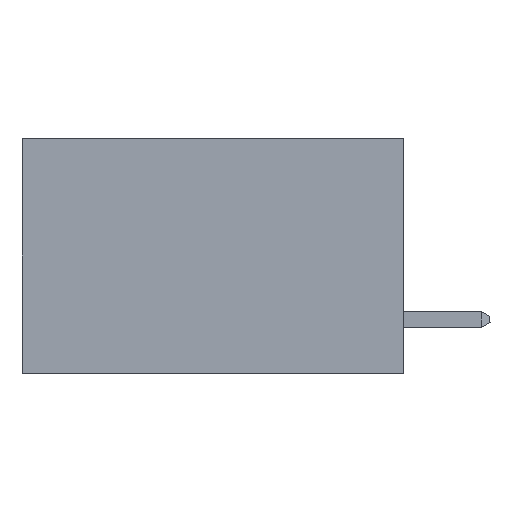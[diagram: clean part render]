
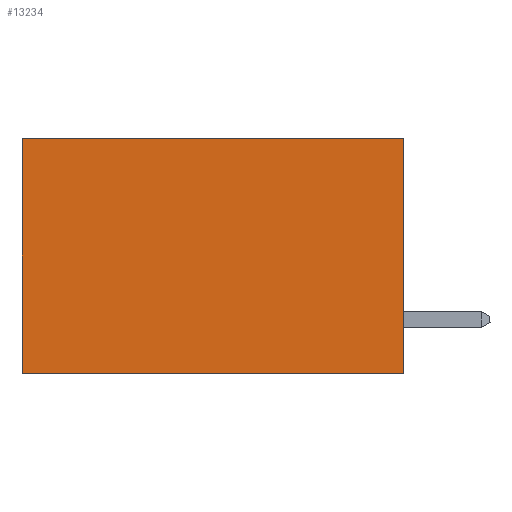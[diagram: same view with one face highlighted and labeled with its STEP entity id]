
A CAD part, left-side view. The second image highlights one B-rep face of the part: STEP entity #13234.
In plain terms, the highlighted planar face has unit normal (-1, 0, 0).
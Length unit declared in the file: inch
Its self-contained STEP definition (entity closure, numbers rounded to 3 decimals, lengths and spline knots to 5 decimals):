
#2181 = VERTEX_POINT ( 'NONE', #15202 ) ;
#2390 = EDGE_CURVE ( 'NONE', #16557, #2181, #4355, .T. ) ;
#2397 = CARTESIAN_POINT ( 'NONE',  ( 0.2875, 0., -0.37 ) ) ;
#2793 = VECTOR ( 'NONE', #9304, 39.37008 ) ;
#3331 = CARTESIAN_POINT ( 'NONE',  ( 0.2875, 0.6, 0. ) ) ;
#4355 = LINE ( 'NONE', #18820, #10524 ) ;
#4847 = EDGE_CURVE ( 'NONE', #10819, #9346, #20010, .T. ) ;
#5075 = ORIENTED_EDGE ( 'NONE', *, *, #2390, .F. ) ;
#5218 = CARTESIAN_POINT ( 'NONE',  ( 0.2875, 0., 0. ) ) ;
#5423 = DIRECTION ( 'NONE',  ( 0., 0., -1. ) ) ;
#5855 = ORIENTED_EDGE ( 'NONE', *, *, #4847, .T. ) ;
#5983 = LINE ( 'NONE', #14081, #16399 ) ;
#8692 = AXIS2_PLACEMENT_3D ( 'NONE', #13256, #14946, #16673 ) ;
#8930 = DIRECTION ( 'NONE',  ( 0., 1., 0. ) ) ;
#9304 = DIRECTION ( 'NONE',  ( 0., 0., -1. ) ) ;
#9346 = VERTEX_POINT ( 'NONE', #3331 ) ;
#9830 = EDGE_CURVE ( 'NONE', #9346, #2181, #20666, .T. ) ;
#10524 = VECTOR ( 'NONE', #15522, 39.37008 ) ;
#10819 = VERTEX_POINT ( 'NONE', #5218 ) ;
#12831 = ORIENTED_EDGE ( 'NONE', *, *, #17840, .F. ) ;
#13234 = ADVANCED_FACE ( 'NONE', ( #19437 ), #21990, .F. ) ;
#13256 = CARTESIAN_POINT ( 'NONE',  ( 0.2875, 0., 0. ) ) ;
#14081 = CARTESIAN_POINT ( 'NONE',  ( 0.2875, 0., 0. ) ) ;
#14424 = CARTESIAN_POINT ( 'NONE',  ( 0.2875, 0.6, 0. ) ) ;
#14946 = DIRECTION ( 'NONE',  ( 1., 0., 0. ) ) ;
#15202 = CARTESIAN_POINT ( 'NONE',  ( 0.2875, 0.6, -0.37 ) ) ;
#15522 = DIRECTION ( 'NONE',  ( 0., 1., 0. ) ) ;
#16399 = VECTOR ( 'NONE', #5423, 39.37008 ) ;
#16557 = VERTEX_POINT ( 'NONE', #2397 ) ;
#16673 = DIRECTION ( 'NONE',  ( 0., 0., -1. ) ) ;
#17376 = VECTOR ( 'NONE', #8930, 39.37008 ) ;
#17840 = EDGE_CURVE ( 'NONE', #10819, #16557, #5983, .T. ) ;
#18168 = ORIENTED_EDGE ( 'NONE', *, *, #9830, .T. ) ;
#18820 = CARTESIAN_POINT ( 'NONE',  ( 0.2875, 0., -0.37 ) ) ;
#19437 = FACE_OUTER_BOUND ( 'NONE', #21064, .T. ) ;
#20010 = LINE ( 'NONE', #20978, #17376 ) ;
#20666 = LINE ( 'NONE', #14424, #2793 ) ;
#20978 = CARTESIAN_POINT ( 'NONE',  ( 0.2875, 0., 0. ) ) ;
#21064 = EDGE_LOOP ( 'NONE', ( #18168, #5075, #12831, #5855 ) ) ;
#21990 = PLANE ( 'NONE',  #8692 ) ;
